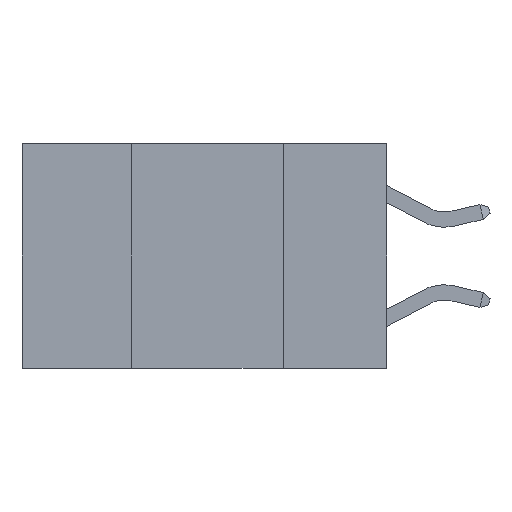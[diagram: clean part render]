
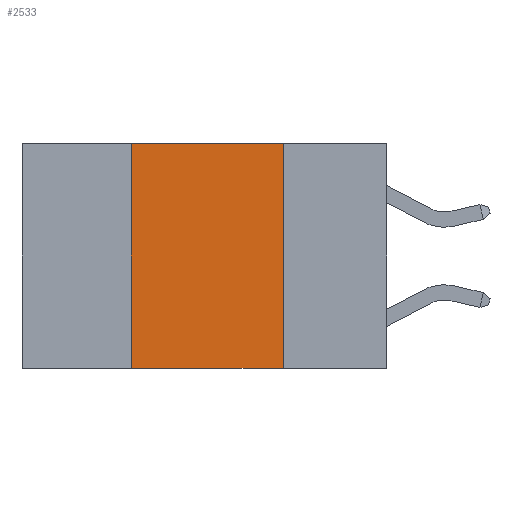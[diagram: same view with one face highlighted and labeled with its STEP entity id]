
A CAD part, left-side view. The second image highlights one B-rep face of the part: STEP entity #2533.
In plain terms, the highlighted planar face has unit normal (-1, 0, 0).
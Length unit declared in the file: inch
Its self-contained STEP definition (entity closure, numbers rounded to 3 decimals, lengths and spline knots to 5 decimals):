
#128 = DIRECTION ( 'NONE',  ( 1., 0., 0. ) ) ;
#214 = DIRECTION ( 'NONE',  ( 0., -1., 0. ) ) ;
#412 = DIRECTION ( 'NONE',  ( 0., 0., -1. ) ) ;
#749 = DIRECTION ( 'NONE',  ( 0., 0., 1. ) ) ;
#959 = VECTOR ( 'NONE', #412, 39.37008 ) ;
#985 = EDGE_CURVE ( 'NONE', #11497, #2212, #12807, .T. ) ;
#1046 = FACE_OUTER_BOUND ( 'NONE', #5113, .T. ) ;
#1614 = EDGE_CURVE ( 'NONE', #11497, #7665, #10640, .T. ) ;
#2047 = DIRECTION ( 'NONE',  ( 0., -1., 0. ) ) ;
#2212 = VERTEX_POINT ( 'NONE', #2532 ) ;
#2532 = CARTESIAN_POINT ( 'NONE',  ( 0., 0.17, -0.37 ) ) ;
#2533 = ADVANCED_FACE ( 'NONE', ( #1046 ), #4211, .F. ) ;
#3022 = CARTESIAN_POINT ( 'NONE',  ( 0., 0.6, -0.37 ) ) ;
#3336 = CARTESIAN_POINT ( 'NONE',  ( 0., 0.6, 0. ) ) ;
#4211 = PLANE ( 'NONE',  #5167 ) ;
#4911 = DIRECTION ( 'NONE',  ( 0., 0., -1. ) ) ;
#5044 = ORIENTED_EDGE ( 'NONE', *, *, #1614, .F. ) ;
#5113 = EDGE_LOOP ( 'NONE', ( #8528, #5454, #5044, #7618 ) ) ;
#5167 = AXIS2_PLACEMENT_3D ( 'NONE', #11065, #128, #4911 ) ;
#5311 = EDGE_CURVE ( 'NONE', #7665, #7805, #8086, .T. ) ;
#5393 = VECTOR ( 'NONE', #2047, 39.37008 ) ;
#5408 = LINE ( 'NONE', #9398, #959 ) ;
#5454 = ORIENTED_EDGE ( 'NONE', *, *, #5311, .F. ) ;
#6214 = CARTESIAN_POINT ( 'NONE',  ( 0., 0.17, 0. ) ) ;
#7618 = ORIENTED_EDGE ( 'NONE', *, *, #985, .T. ) ;
#7665 = VERTEX_POINT ( 'NONE', #12359 ) ;
#7805 = VERTEX_POINT ( 'NONE', #6214 ) ;
#8086 = LINE ( 'NONE', #3336, #10015 ) ;
#8405 = EDGE_CURVE ( 'NONE', #7805, #2212, #5408, .T. ) ;
#8528 = ORIENTED_EDGE ( 'NONE', *, *, #8405, .F. ) ;
#9398 = CARTESIAN_POINT ( 'NONE',  ( 0., 0.17, 0. ) ) ;
#10015 = VECTOR ( 'NONE', #214, 39.37008 ) ;
#10367 = VECTOR ( 'NONE', #749, 39.37008 ) ;
#10640 = LINE ( 'NONE', #10705, #10367 ) ;
#10705 = CARTESIAN_POINT ( 'NONE',  ( 0., 0.42, 0. ) ) ;
#10975 = CARTESIAN_POINT ( 'NONE',  ( 0., 0.42, -0.37 ) ) ;
#11065 = CARTESIAN_POINT ( 'NONE',  ( 0., 0.6, 0. ) ) ;
#11497 = VERTEX_POINT ( 'NONE', #10975 ) ;
#12359 = CARTESIAN_POINT ( 'NONE',  ( 0., 0.42, 0. ) ) ;
#12807 = LINE ( 'NONE', #3022, #5393 ) ;
